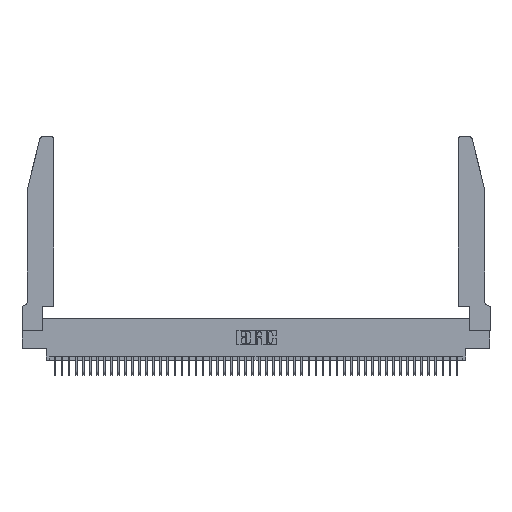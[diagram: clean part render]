
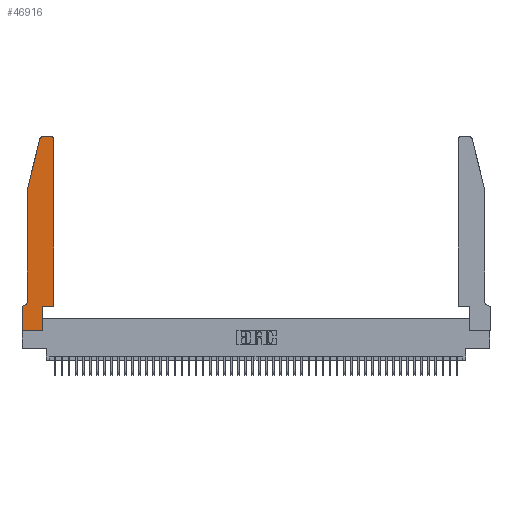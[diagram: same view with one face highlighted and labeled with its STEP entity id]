
A CAD part, top view. The second image highlights one B-rep face of the part: STEP entity #46916.
In plain terms, the highlighted planar face has unit normal (0, 0, 1).
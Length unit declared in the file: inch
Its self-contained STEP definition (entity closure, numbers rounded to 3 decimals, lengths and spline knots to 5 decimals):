
#610 = FACE_OUTER_BOUND ( 'NONE', #5733, .T. ) ;
#784 = LINE ( 'NONE', #30570, #28061 ) ;
#1198 = DIRECTION ( 'NONE',  ( -1., 0., 0. ) ) ;
#1852 = EDGE_CURVE ( 'NONE', #2627, #30962, #9554, .T. ) ;
#1999 = EDGE_CURVE ( 'NONE', #30962, #22637, #14447, .T. ) ;
#2101 = CIRCLE ( 'NONE', #43142, 0.03 ) ;
#2461 = CARTESIAN_POINT ( 'NONE',  ( 0.4505, 2.72, 0.37 ) ) ;
#2627 = VERTEX_POINT ( 'NONE', #42652 ) ;
#2684 = CARTESIAN_POINT ( 'NONE',  ( 0.0055, 0.42, 0.37 ) ) ;
#2819 = VERTEX_POINT ( 'NONE', #17269 ) ;
#2962 = DIRECTION ( 'NONE',  ( -0.239, -0.971, 0. ) ) ;
#4077 = VERTEX_POINT ( 'NONE', #34793 ) ;
#4328 = EDGE_CURVE ( 'NONE', #5202, #14435, #784, .T. ) ;
#5202 = VERTEX_POINT ( 'NONE', #30285 ) ;
#5311 = CARTESIAN_POINT ( 'NONE',  ( 0.4505, 0.35, 0.37 ) ) ;
#5319 = AXIS2_PLACEMENT_3D ( 'NONE', #2684, #13949, #10505 ) ;
#5328 = CARTESIAN_POINT ( 'NONE',  ( 0., 0., 0.37 ) ) ;
#5343 = CARTESIAN_POINT ( 'NONE',  ( 0.0755, 2., 0.37 ) ) ;
#5733 = EDGE_LOOP ( 'NONE', ( #15398, #18404, #21638, #6058, #38739, #36849, #25066, #34506, #27287, #44690, #30590, #31086 ) ) ;
#5935 = LINE ( 'NONE', #39796, #42780 ) ;
#6058 = ORIENTED_EDGE ( 'NONE', *, *, #6319, .T. ) ;
#6319 = EDGE_CURVE ( 'NONE', #14435, #47470, #13711, .T. ) ;
#6418 = VERTEX_POINT ( 'NONE', #2461 ) ;
#8160 = DIRECTION ( 'NONE',  ( 0., 0., 1. ) ) ;
#9554 = LINE ( 'NONE', #32190, #24728 ) ;
#10505 = DIRECTION ( 'NONE',  ( -1., 0., 0. ) ) ;
#10693 = EDGE_CURVE ( 'NONE', #22637, #2819, #22891, .T. ) ;
#13066 = VECTOR ( 'NONE', #25731, 39.37008 ) ;
#13189 = EDGE_CURVE ( 'NONE', #6418, #40613, #36648, .T. ) ;
#13711 = LINE ( 'NONE', #40893, #13066 ) ;
#13949 = DIRECTION ( 'NONE',  ( 0., 0., -1. ) ) ;
#14340 = CARTESIAN_POINT ( 'NONE',  ( 0.4505, 0.35, 0.37 ) ) ;
#14435 = VERTEX_POINT ( 'NONE', #5343 ) ;
#14447 = LINE ( 'NONE', #40332, #26470 ) ;
#14793 = CIRCLE ( 'NONE', #5319, 0.07 ) ;
#15398 = ORIENTED_EDGE ( 'NONE', *, *, #48274, .T. ) ;
#16769 = DIRECTION ( 'NONE',  ( -1., 0., 0. ) ) ;
#17269 = CARTESIAN_POINT ( 'NONE',  ( 0.2865, 0., 0.37 ) ) ;
#18245 = DIRECTION ( 'NONE',  ( 1., 0., 0. ) ) ;
#18404 = ORIENTED_EDGE ( 'NONE', *, *, #19927, .T. ) ;
#19674 = LINE ( 'NONE', #14340, #35985 ) ;
#19694 = DIRECTION ( 'NONE',  ( 1., 0., 0. ) ) ;
#19708 = EDGE_CURVE ( 'NONE', #4077, #6418, #31845, .T. ) ;
#19927 = EDGE_CURVE ( 'NONE', #37612, #5202, #2101, .T. ) ;
#21638 = ORIENTED_EDGE ( 'NONE', *, *, #4328, .T. ) ;
#21965 = AXIS2_PLACEMENT_3D ( 'NONE', #39711, #46911, #19694 ) ;
#22637 = VERTEX_POINT ( 'NONE', #5328 ) ;
#22891 = LINE ( 'NONE', #39830, #38534 ) ;
#24490 = DIRECTION ( 'NONE',  ( 0., 0., 1. ) ) ;
#24728 = VECTOR ( 'NONE', #1198, 39.37008 ) ;
#25066 = ORIENTED_EDGE ( 'NONE', *, *, #1999, .T. ) ;
#25731 = DIRECTION ( 'NONE',  ( 0., -1., 0. ) ) ;
#26470 = VECTOR ( 'NONE', #47372, 39.37008 ) ;
#27287 = ORIENTED_EDGE ( 'NONE', *, *, #48046, .T. ) ;
#28061 = VECTOR ( 'NONE', #2962, 39.37008 ) ;
#29552 = LINE ( 'NONE', #34257, #30176 ) ;
#30176 = VECTOR ( 'NONE', #45496, 39.37008 ) ;
#30285 = CARTESIAN_POINT ( 'NONE',  ( 0.25487, 2.72718, 0.37 ) ) ;
#30429 = CARTESIAN_POINT ( 'NONE',  ( 0.0755, 0.42, 0.37 ) ) ;
#30570 = CARTESIAN_POINT ( 'NONE',  ( 0.0755, 2., 0.37 ) ) ;
#30590 = ORIENTED_EDGE ( 'NONE', *, *, #19708, .T. ) ;
#30962 = VERTEX_POINT ( 'NONE', #42009 ) ;
#31004 = CARTESIAN_POINT ( 'NONE',  ( 0., 0.35, 0.37 ) ) ;
#31086 = ORIENTED_EDGE ( 'NONE', *, *, #13189, .T. ) ;
#31625 = DIRECTION ( 'NONE',  ( 1., 0., 0. ) ) ;
#31845 = LINE ( 'NONE', #5311, #39032 ) ;
#32031 = CARTESIAN_POINT ( 'NONE',  ( 0.284, 2.72, 0.37 ) ) ;
#32190 = CARTESIAN_POINT ( 'NONE',  ( 0.0755, 0.35, 0.37 ) ) ;
#34257 = CARTESIAN_POINT ( 'NONE',  ( 0.2865, 0.35, 0.37 ) ) ;
#34471 = CARTESIAN_POINT ( 'NONE',  ( 0.4205, 2.75, 0.37 ) ) ;
#34506 = ORIENTED_EDGE ( 'NONE', *, *, #10693, .T. ) ;
#34718 = PLANE ( 'NONE',  #45758 ) ;
#34793 = CARTESIAN_POINT ( 'NONE',  ( 0.4505, 0.35, 0.37 ) ) ;
#35046 = CARTESIAN_POINT ( 'NONE',  ( 0.284, 2.75, 0.37 ) ) ;
#35985 = VECTOR ( 'NONE', #18245, 39.37008 ) ;
#36648 = CIRCLE ( 'NONE', #21965, 0.03 ) ;
#36849 = ORIENTED_EDGE ( 'NONE', *, *, #1852, .T. ) ;
#37612 = VERTEX_POINT ( 'NONE', #35046 ) ;
#38534 = VECTOR ( 'NONE', #31625, 39.37008 ) ;
#38739 = ORIENTED_EDGE ( 'NONE', *, *, #44320, .T. ) ;
#39032 = VECTOR ( 'NONE', #45841, 39.37008 ) ;
#39711 = CARTESIAN_POINT ( 'NONE',  ( 0.4205, 2.72, 0.37 ) ) ;
#39796 = CARTESIAN_POINT ( 'NONE',  ( 0.2605, 2.75, 0.37 ) ) ;
#39830 = CARTESIAN_POINT ( 'NONE',  ( 0., 0., 0.37 ) ) ;
#40332 = CARTESIAN_POINT ( 'NONE',  ( 0., 0., 0.37 ) ) ;
#40613 = VERTEX_POINT ( 'NONE', #34471 ) ;
#40893 = CARTESIAN_POINT ( 'NONE',  ( 0.0755, 2., 0.37 ) ) ;
#42009 = CARTESIAN_POINT ( 'NONE',  ( 0., 0.35, 0.37 ) ) ;
#42577 = DIRECTION ( 'NONE',  ( 1., 0., 0. ) ) ;
#42652 = CARTESIAN_POINT ( 'NONE',  ( 0.0055, 0.35, 0.37 ) ) ;
#42780 = VECTOR ( 'NONE', #16769, 39.37008 ) ;
#43082 = VERTEX_POINT ( 'NONE', #43413 ) ;
#43142 = AXIS2_PLACEMENT_3D ( 'NONE', #32031, #24490, #44134 ) ;
#43413 = CARTESIAN_POINT ( 'NONE',  ( 0.2865, 0.35, 0.37 ) ) ;
#44134 = DIRECTION ( 'NONE',  ( 1., 0., 0. ) ) ;
#44320 = EDGE_CURVE ( 'NONE', #47470, #2627, #14793, .T. ) ;
#44690 = ORIENTED_EDGE ( 'NONE', *, *, #44775, .T. ) ;
#44775 = EDGE_CURVE ( 'NONE', #43082, #4077, #19674, .T. ) ;
#45496 = DIRECTION ( 'NONE',  ( 0., 1., 0. ) ) ;
#45758 = AXIS2_PLACEMENT_3D ( 'NONE', #31004, #8160, #42577 ) ;
#45841 = DIRECTION ( 'NONE',  ( 0., 1., 0. ) ) ;
#46911 = DIRECTION ( 'NONE',  ( 0., 0., 1. ) ) ;
#46916 = ADVANCED_FACE ( 'NONE', ( #610 ), #34718, .T. ) ;
#47372 = DIRECTION ( 'NONE',  ( 0., -1., 0. ) ) ;
#47470 = VERTEX_POINT ( 'NONE', #30429 ) ;
#48046 = EDGE_CURVE ( 'NONE', #2819, #43082, #29552, .T. ) ;
#48274 = EDGE_CURVE ( 'NONE', #40613, #37612, #5935, .T. ) ;
